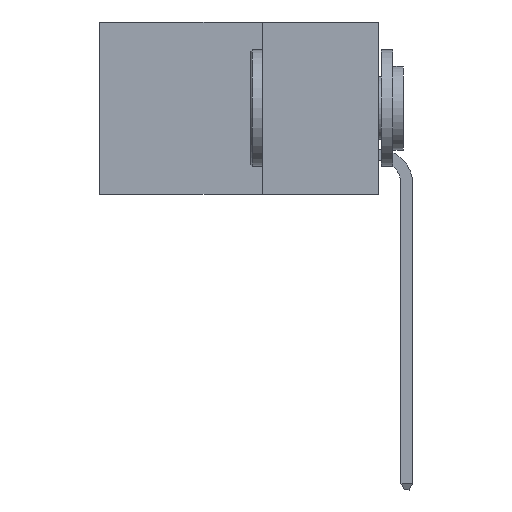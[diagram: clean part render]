
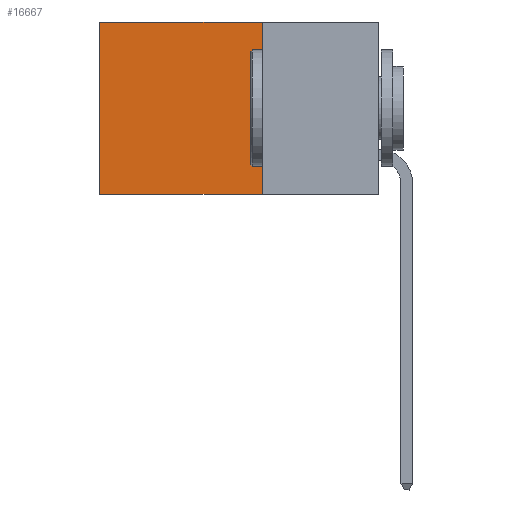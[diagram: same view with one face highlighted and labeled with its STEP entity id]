
A CAD part, left-side view. The second image highlights one B-rep face of the part: STEP entity #16667.
In plain terms, the highlighted planar face has unit normal (-1, 0, 0).
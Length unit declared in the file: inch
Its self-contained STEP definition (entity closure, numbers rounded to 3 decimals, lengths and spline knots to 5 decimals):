
#618 = CARTESIAN_POINT ( 'NONE',  ( 0.298, 0.6, 0. ) ) ;
#1260 = DIRECTION ( 'NONE',  ( 1., 0., 0. ) ) ;
#2575 = EDGE_CURVE ( 'NONE', #17515, #9107, #7001, .T. ) ;
#2734 = CARTESIAN_POINT ( 'NONE',  ( 0.298, 0.6, 0. ) ) ;
#2818 = VECTOR ( 'NONE', #16553, 39.37008 ) ;
#3038 = DIRECTION ( 'NONE',  ( 0., 0., -1. ) ) ;
#3300 = EDGE_LOOP ( 'NONE', ( #10090, #8546, #9447, #7415 ) ) ;
#4033 = DIRECTION ( 'NONE',  ( 0., 1., 0. ) ) ;
#4124 = EDGE_CURVE ( 'NONE', #17515, #14149, #5867, .T. ) ;
#4662 = LINE ( 'NONE', #618, #7949 ) ;
#4956 = CARTESIAN_POINT ( 'NONE',  ( 0.298, 0.25, -0.37 ) ) ;
#5867 = LINE ( 'NONE', #18212, #16754 ) ;
#6933 = VECTOR ( 'NONE', #4033, 39.37008 ) ;
#7001 = LINE ( 'NONE', #12438, #2818 ) ;
#7415 = ORIENTED_EDGE ( 'NONE', *, *, #2575, .T. ) ;
#7418 = CARTESIAN_POINT ( 'NONE',  ( 0.298, 0.25, 0. ) ) ;
#7796 = FACE_OUTER_BOUND ( 'NONE', #3300, .T. ) ;
#7949 = VECTOR ( 'NONE', #12163, 39.37008 ) ;
#8235 = CARTESIAN_POINT ( 'NONE',  ( 0.298, 0.25, -0.37 ) ) ;
#8398 = PLANE ( 'NONE',  #12914 ) ;
#8546 = ORIENTED_EDGE ( 'NONE', *, *, #15830, .F. ) ;
#9107 = VERTEX_POINT ( 'NONE', #2734 ) ;
#9447 = ORIENTED_EDGE ( 'NONE', *, *, #4124, .F. ) ;
#10090 = ORIENTED_EDGE ( 'NONE', *, *, #12260, .T. ) ;
#11308 = DIRECTION ( 'NONE',  ( 0., 0., -1. ) ) ;
#11859 = CARTESIAN_POINT ( 'NONE',  ( 0.298, 0.6, -0.37 ) ) ;
#12163 = DIRECTION ( 'NONE',  ( 0., 0., -1. ) ) ;
#12260 = EDGE_CURVE ( 'NONE', #9107, #17571, #4662, .T. ) ;
#12438 = CARTESIAN_POINT ( 'NONE',  ( 0.298, 0.25, 0. ) ) ;
#12914 = AXIS2_PLACEMENT_3D ( 'NONE', #18285, #1260, #11308 ) ;
#14149 = VERTEX_POINT ( 'NONE', #4956 ) ;
#15830 = EDGE_CURVE ( 'NONE', #14149, #17571, #18251, .T. ) ;
#16553 = DIRECTION ( 'NONE',  ( 0., 1., 0. ) ) ;
#16667 = ADVANCED_FACE ( 'NONE', ( #7796 ), #8398, .F. ) ;
#16754 = VECTOR ( 'NONE', #3038, 39.37008 ) ;
#17515 = VERTEX_POINT ( 'NONE', #7418 ) ;
#17571 = VERTEX_POINT ( 'NONE', #11859 ) ;
#18212 = CARTESIAN_POINT ( 'NONE',  ( 0.298, 0.25, 0. ) ) ;
#18251 = LINE ( 'NONE', #8235, #6933 ) ;
#18285 = CARTESIAN_POINT ( 'NONE',  ( 0.298, 0.25, 0. ) ) ;
